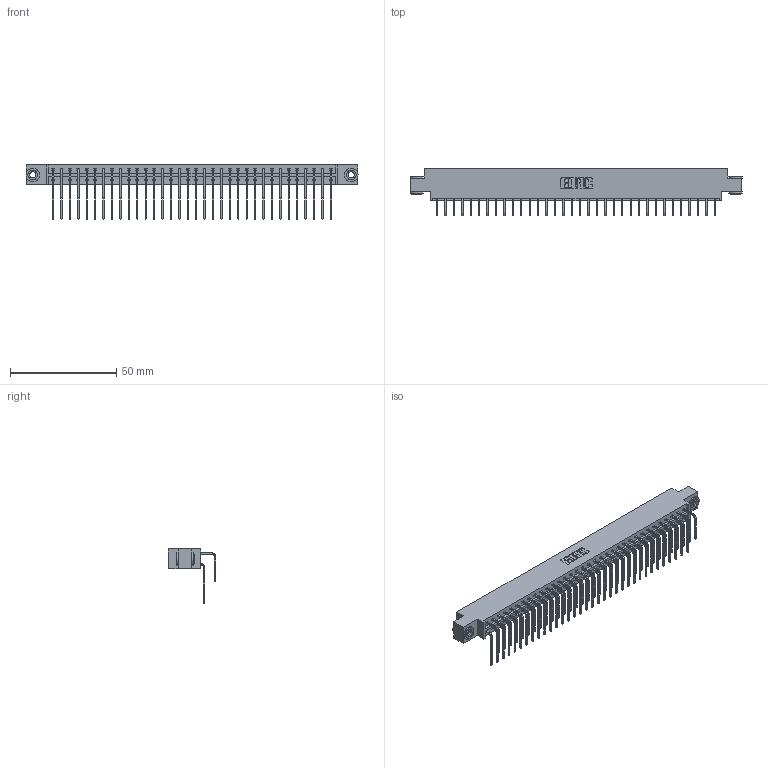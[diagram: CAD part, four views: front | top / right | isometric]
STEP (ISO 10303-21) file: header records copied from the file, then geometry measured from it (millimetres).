
FILE_DESCRIPTION (( 'STEP AP203' ), '1' );
FILE_NAME ('833-068-558-803.STEP', '2020-06-05T11:22:35', ( '' ), ( '' ), 'SwSTEP 2.0', 'SolidWorks 2020', '' );
FILE_SCHEMA (( 'CONFIG_CONTROL_DESIGN' ));
Length unit declared in the file: inch
Products named in the file (5): 345-292-001_558 559 Tail - 1; 833-068-558-803; 345-292-001_558 Tail - 2; 345-250-002_345-250-002-102; 833 Part_Offset - .156 Dia - TH
Assembly tree (71 placements, depth 2):
  833-068-558-803
    833 Part_Offset - .156 Dia - TH
    345-292-001_558 559 Tail - 1  x34
    345-292-001_558 Tail - 2  x34
    345-250-002_345-250-002-102  x2
Bounding box: 156.26 x 22.17 x 25.53 mm (x, y, z)
Volume: 16062.4 mm3; surface area: 21299.4 mm2
Topology: 71 solids, 71 shells, 3828 faces, 11347 edges, 7470 vertices
Faces by surface type: plane 2668, cylinder 1152, cone 8
Entity records: 25474 total; most frequent: CARTESIAN_POINT 4260, ORIENTED_EDGE 4138, DIRECTION 3667, EDGE_CURVE 2069, LINE 1877, VECTOR 1877, VERTEX_POINT 1374, AXIS2_PLACEMENT_3D 895
